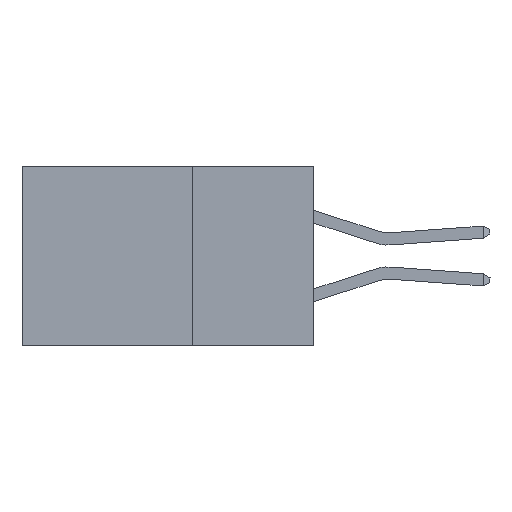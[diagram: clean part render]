
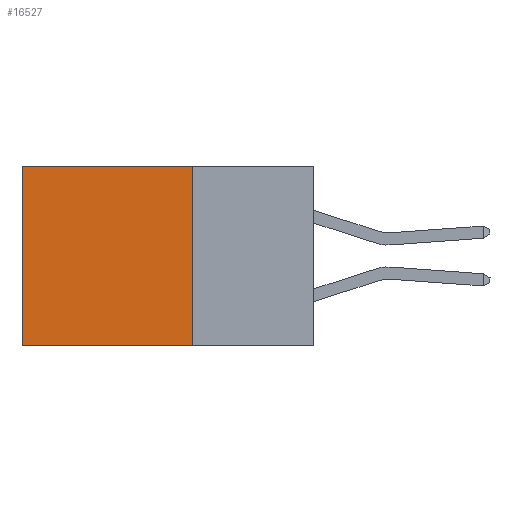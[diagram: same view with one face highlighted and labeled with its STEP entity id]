
A CAD part, left-side view. The second image highlights one B-rep face of the part: STEP entity #16527.
In plain terms, the highlighted planar face has unit normal (-1, 0, 0).
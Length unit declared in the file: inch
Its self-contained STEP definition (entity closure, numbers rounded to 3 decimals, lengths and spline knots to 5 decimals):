
#89 = LINE ( 'NONE', #7655, #3756 ) ;
#800 = VECTOR ( 'NONE', #7790, 39.37008 ) ;
#1883 = ORIENTED_EDGE ( 'NONE', *, *, #11014, .F. ) ;
#2452 = VERTEX_POINT ( 'NONE', #5162 ) ;
#3513 = VERTEX_POINT ( 'NONE', #8268 ) ;
#3756 = VECTOR ( 'NONE', #7722, 39.37008 ) ;
#4202 = CARTESIAN_POINT ( 'NONE',  ( 0.2875, 0.25, 0. ) ) ;
#5162 = CARTESIAN_POINT ( 'NONE',  ( 0.2875, 0.6, -0.37 ) ) ;
#5735 = DIRECTION ( 'NONE',  ( 1., 0., 0. ) ) ;
#6055 = CARTESIAN_POINT ( 'NONE',  ( 0.2875, 0.25, -0.37 ) ) ;
#6232 = CARTESIAN_POINT ( 'NONE',  ( 0.2875, 0.25, 0. ) ) ;
#7427 = LINE ( 'NONE', #16310, #14677 ) ;
#7655 = CARTESIAN_POINT ( 'NONE',  ( 0.2875, 0.25, -0.37 ) ) ;
#7722 = DIRECTION ( 'NONE',  ( 0., 1., 0. ) ) ;
#7785 = LINE ( 'NONE', #8862, #19171 ) ;
#7790 = DIRECTION ( 'NONE',  ( 0., 1., 0. ) ) ;
#8188 = EDGE_LOOP ( 'NONE', ( #15021, #1883, #13290, #12662 ) ) ;
#8268 = CARTESIAN_POINT ( 'NONE',  ( 0.2875, 0.25, 0. ) ) ;
#8717 = VERTEX_POINT ( 'NONE', #14563 ) ;
#8862 = CARTESIAN_POINT ( 'NONE',  ( 0.2875, 0.6, 0. ) ) ;
#10428 = DIRECTION ( 'NONE',  ( 0., 0., -1. ) ) ;
#11014 = EDGE_CURVE ( 'NONE', #17204, #2452, #89, .T. ) ;
#11690 = DIRECTION ( 'NONE',  ( 0., 0., -1. ) ) ;
#12662 = ORIENTED_EDGE ( 'NONE', *, *, #19290, .T. ) ;
#13191 = LINE ( 'NONE', #6232, #800 ) ;
#13290 = ORIENTED_EDGE ( 'NONE', *, *, #18296, .F. ) ;
#13449 = PLANE ( 'NONE',  #18654 ) ;
#14563 = CARTESIAN_POINT ( 'NONE',  ( 0.2875, 0.6, 0. ) ) ;
#14625 = EDGE_CURVE ( 'NONE', #8717, #2452, #7785, .T. ) ;
#14677 = VECTOR ( 'NONE', #11690, 39.37008 ) ;
#14761 = FACE_OUTER_BOUND ( 'NONE', #8188, .T. ) ;
#15021 = ORIENTED_EDGE ( 'NONE', *, *, #14625, .T. ) ;
#16310 = CARTESIAN_POINT ( 'NONE',  ( 0.2875, 0.25, 0. ) ) ;
#16527 = ADVANCED_FACE ( 'NONE', ( #14761 ), #13449, .F. ) ;
#16586 = DIRECTION ( 'NONE',  ( 0., 0., -1. ) ) ;
#17204 = VERTEX_POINT ( 'NONE', #6055 ) ;
#18296 = EDGE_CURVE ( 'NONE', #3513, #17204, #7427, .T. ) ;
#18654 = AXIS2_PLACEMENT_3D ( 'NONE', #4202, #5735, #16586 ) ;
#19171 = VECTOR ( 'NONE', #10428, 39.37008 ) ;
#19290 = EDGE_CURVE ( 'NONE', #3513, #8717, #13191, .T. ) ;
